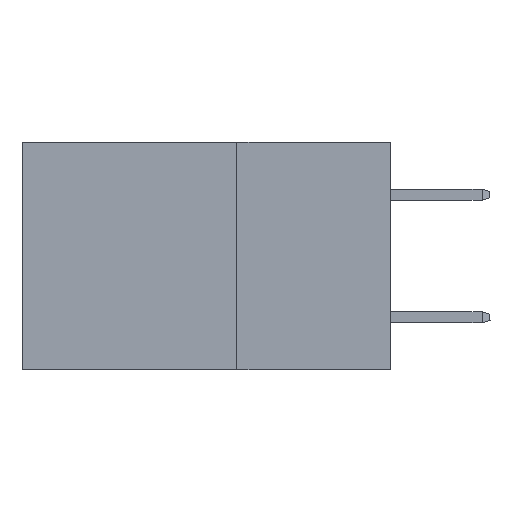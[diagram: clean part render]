
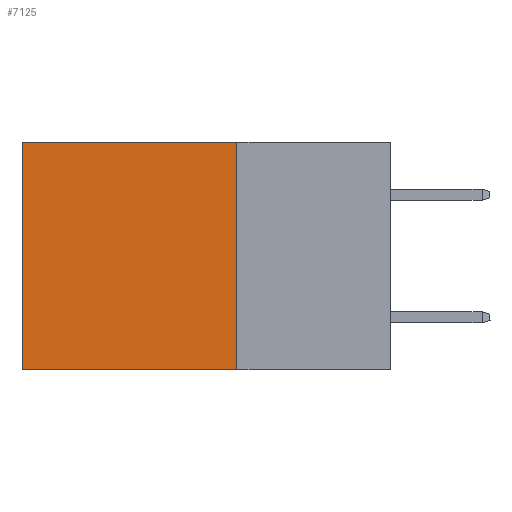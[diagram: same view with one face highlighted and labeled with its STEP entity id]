
A CAD part, left-side view. The second image highlights one B-rep face of the part: STEP entity #7125.
In plain terms, the highlighted planar face has unit normal (-1, 0, 0).
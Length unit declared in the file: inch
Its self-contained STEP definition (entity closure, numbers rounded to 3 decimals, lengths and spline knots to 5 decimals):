
#269 = VECTOR ( 'NONE', #15940, 39.37008 ) ;
#2262 = ORIENTED_EDGE ( 'NONE', *, *, #21884, .F. ) ;
#4291 = DIRECTION ( 'NONE',  ( 0., 0., -1. ) ) ;
#4613 = VECTOR ( 'NONE', #14819, 39.37008 ) ;
#4990 = EDGE_CURVE ( 'NONE', #25604, #41422, #25272, .T. ) ;
#5973 = CARTESIAN_POINT ( 'NONE',  ( 0.2875, 0.6, 0. ) ) ;
#7125 = ADVANCED_FACE ( 'NONE', ( #17353 ), #27121, .F. ) ;
#7676 = VERTEX_POINT ( 'NONE', #27900 ) ;
#8469 = ORIENTED_EDGE ( 'NONE', *, *, #27348, .F. ) ;
#12437 = EDGE_LOOP ( 'NONE', ( #39809, #2262, #8469, #41728 ) ) ;
#12857 = CARTESIAN_POINT ( 'NONE',  ( 0.2875, 0.25, 0. ) ) ;
#14456 = LINE ( 'NONE', #24410, #20207 ) ;
#14819 = DIRECTION ( 'NONE',  ( 0., 1., 0. ) ) ;
#15940 = DIRECTION ( 'NONE',  ( 0., 0., -1. ) ) ;
#17152 = EDGE_CURVE ( 'NONE', #7676, #25604, #34364, .T. ) ;
#17353 = FACE_OUTER_BOUND ( 'NONE', #12437, .T. ) ;
#19429 = DIRECTION ( 'NONE',  ( 0., 1., 0. ) ) ;
#20053 = LINE ( 'NONE', #29420, #25760 ) ;
#20207 = VECTOR ( 'NONE', #4291, 39.37008 ) ;
#21884 = EDGE_CURVE ( 'NONE', #29246, #41422, #20053, .T. ) ;
#23627 = CARTESIAN_POINT ( 'NONE',  ( 0.2875, 0.6, 0. ) ) ;
#24410 = CARTESIAN_POINT ( 'NONE',  ( 0.2875, 0.25, 0. ) ) ;
#25272 = LINE ( 'NONE', #5973, #269 ) ;
#25604 = VERTEX_POINT ( 'NONE', #23627 ) ;
#25760 = VECTOR ( 'NONE', #19429, 39.37008 ) ;
#27121 = PLANE ( 'NONE',  #39721 ) ;
#27348 = EDGE_CURVE ( 'NONE', #7676, #29246, #14456, .T. ) ;
#27900 = CARTESIAN_POINT ( 'NONE',  ( 0.2875, 0.25, 0. ) ) ;
#27950 = CARTESIAN_POINT ( 'NONE',  ( 0.2875, 0.25, 0. ) ) ;
#28614 = CARTESIAN_POINT ( 'NONE',  ( 0.2875, 0.25, -0.37 ) ) ;
#29246 = VERTEX_POINT ( 'NONE', #28614 ) ;
#29420 = CARTESIAN_POINT ( 'NONE',  ( 0.2875, 0.25, -0.37 ) ) ;
#29974 = CARTESIAN_POINT ( 'NONE',  ( 0.2875, 0.6, -0.37 ) ) ;
#34364 = LINE ( 'NONE', #12857, #4613 ) ;
#39721 = AXIS2_PLACEMENT_3D ( 'NONE', #27950, #40081, #40919 ) ;
#39809 = ORIENTED_EDGE ( 'NONE', *, *, #4990, .T. ) ;
#40081 = DIRECTION ( 'NONE',  ( 1., 0., 0. ) ) ;
#40919 = DIRECTION ( 'NONE',  ( 0., 0., -1. ) ) ;
#41422 = VERTEX_POINT ( 'NONE', #29974 ) ;
#41728 = ORIENTED_EDGE ( 'NONE', *, *, #17152, .T. ) ;
